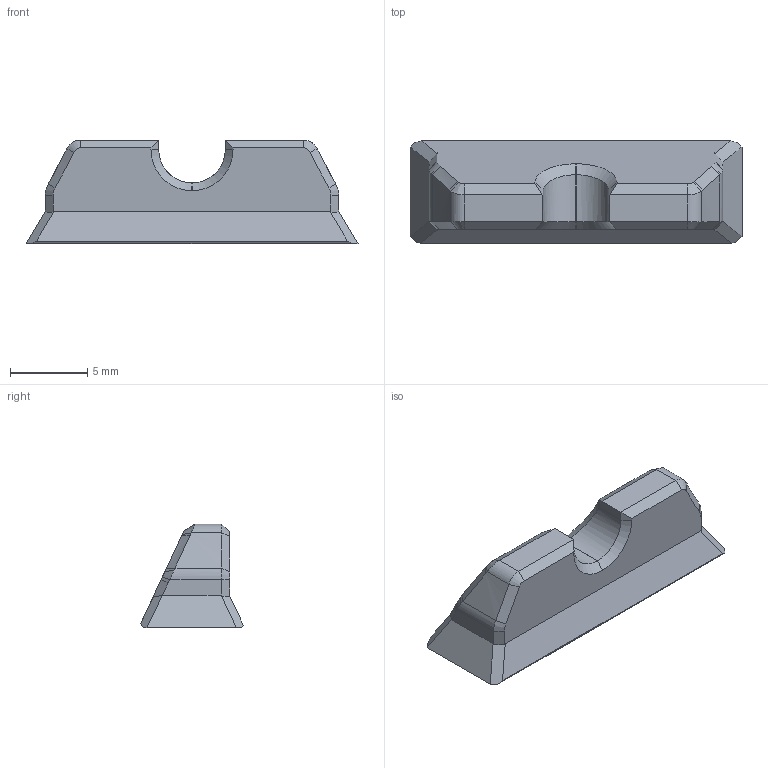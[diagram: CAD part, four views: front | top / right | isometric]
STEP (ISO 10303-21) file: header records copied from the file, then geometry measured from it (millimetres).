
FILE_DESCRIPTION(/* description */ (''),/* implementation_level */ '2;1');
FILE_NAME(/* name */ 'U Notch 6.5 Rear Sight.step',/* time_stamp */ '2021-03-12T12:36:29-05:00',/* author */ (''),/* organization */ (''),/* preprocessor_version */ 'ST-DEVELOPER v18.1',/* originating_system */ 'Autodesk Translation Framework v9.10.0.1330',/* authorisation */ '');
FILE_SCHEMA (('AUTOMOTIVE_DESIGN { 1 0 10303 214 3 1 1 }'));
Length unit declared in the file: millimetre
Products named in the file (1): U Notch 6.5 Rear Sight
Bounding box: 21.5 x 6.65 x 6.72 mm (x, y, z)
Volume: 525.6 mm3; surface area: 491 mm2
Topology: 1 solids, 1 shells, 65 faces, 163 edges, 100 vertices
Faces by surface type: plane 33, bspline 16, cone 8, cylinder 8
Entity records: 2177 total; most frequent: CARTESIAN_POINT 697, ORIENTED_EDGE 326, DIRECTION 245, EDGE_CURVE 163, LINE 113, VECTOR 113, VERTEX_POINT 100, AXIS2_PLACEMENT_3D 66
